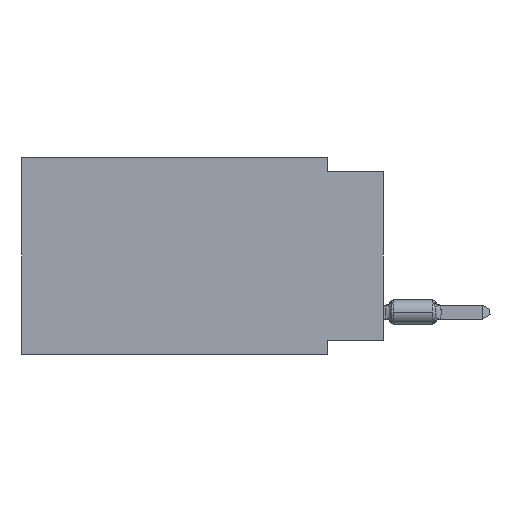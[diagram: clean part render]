
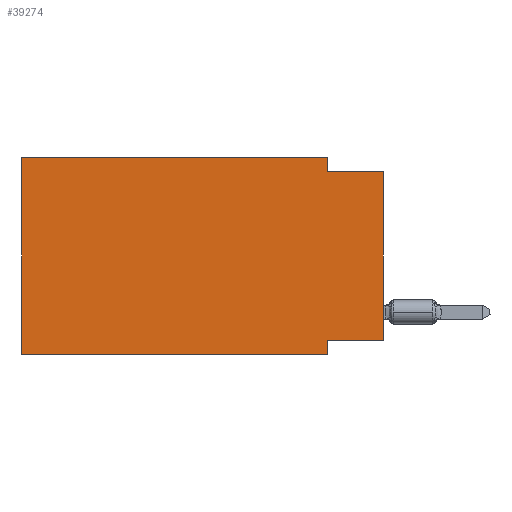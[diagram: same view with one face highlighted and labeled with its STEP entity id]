
A CAD part, left-side view. The second image highlights one B-rep face of the part: STEP entity #39274.
In plain terms, the highlighted planar face has unit normal (-1, 0, 0).
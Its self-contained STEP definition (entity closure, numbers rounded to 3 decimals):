
#858 = ORIENTED_EDGE ( 'NONE', *, *, #37214, .F. ) ;
#1482 = DIRECTION ( 'NONE',  ( 0., 0., 1. ) ) ;
#1789 = CARTESIAN_POINT ( 'NONE',  ( 0., 16.383, 0. ) ) ;
#6985 = EDGE_CURVE ( 'NONE', #53884, #17438, #54228, .T. ) ;
#7641 = VERTEX_POINT ( 'NONE', #52928 ) ;
#9204 = CARTESIAN_POINT ( 'NONE',  ( 0., 0., -8.255 ) ) ;
#9885 = VERTEX_POINT ( 'NONE', #91576 ) ;
#10788 = LINE ( 'NONE', #63070, #44909 ) ;
#12004 = ORIENTED_EDGE ( 'NONE', *, *, #6985, .T. ) ;
#13472 = EDGE_CURVE ( 'NONE', #9885, #17438, #38444, .T. ) ;
#17182 = CARTESIAN_POINT ( 'NONE',  ( 0., 0., -8.255 ) ) ;
#17438 = VERTEX_POINT ( 'NONE', #84281 ) ;
#18834 = CARTESIAN_POINT ( 'NONE',  ( 0., 2.54, -8.89 ) ) ;
#19425 = EDGE_CURVE ( 'NONE', #7641, #9885, #79065, .T. ) ;
#19541 = VERTEX_POINT ( 'NONE', #66823 ) ;
#25354 = FACE_OUTER_BOUND ( 'NONE', #63325, .T. ) ;
#25574 = VECTOR ( 'NONE', #54132, 1000. ) ;
#25694 = CARTESIAN_POINT ( 'NONE',  ( 0., 2.54, -8.255 ) ) ;
#26208 = VECTOR ( 'NONE', #48647, 1000. ) ;
#26300 = ORIENTED_EDGE ( 'NONE', *, *, #95057, .F. ) ;
#26373 = VECTOR ( 'NONE', #78583, 1000. ) ;
#27062 = VECTOR ( 'NONE', #63108, 1000. ) ;
#27740 = CARTESIAN_POINT ( 'NONE',  ( 0., 2.54, 0. ) ) ;
#28400 = EDGE_CURVE ( 'NONE', #70305, #19541, #86717, .T. ) ;
#31174 = LINE ( 'NONE', #67833, #25574 ) ;
#31264 = ORIENTED_EDGE ( 'NONE', *, *, #28400, .F. ) ;
#31972 = ORIENTED_EDGE ( 'NONE', *, *, #13472, .F. ) ;
#33041 = LINE ( 'NONE', #1789, #46982 ) ;
#34318 = VERTEX_POINT ( 'NONE', #50012 ) ;
#37214 = EDGE_CURVE ( 'NONE', #53884, #70305, #84121, .T. ) ;
#38444 = LINE ( 'NONE', #54068, #39547 ) ;
#39274 = ADVANCED_FACE ( 'NONE', ( #25354 ), #60589, .F. ) ;
#39547 = VECTOR ( 'NONE', #47225, 1000. ) ;
#40606 = DIRECTION ( 'NONE',  ( 0., -1., 0. ) ) ;
#42640 = VECTOR ( 'NONE', #1482, 1000. ) ;
#44909 = VECTOR ( 'NONE', #40606, 1000. ) ;
#46982 = VECTOR ( 'NONE', #53563, 1000. ) ;
#47225 = DIRECTION ( 'NONE',  ( 0., -1., 0. ) ) ;
#48647 = DIRECTION ( 'NONE',  ( 0., 0., -1. ) ) ;
#50012 = CARTESIAN_POINT ( 'NONE',  ( 0., 16.383, -8.89 ) ) ;
#50145 = VERTEX_POINT ( 'NONE', #72106 ) ;
#52928 = CARTESIAN_POINT ( 'NONE',  ( 0., 2.54, 0. ) ) ;
#53563 = DIRECTION ( 'NONE',  ( 0., 0., 1. ) ) ;
#53884 = VERTEX_POINT ( 'NONE', #9204 ) ;
#54068 = CARTESIAN_POINT ( 'NONE',  ( 0., 0., -0.635 ) ) ;
#54132 = DIRECTION ( 'NONE',  ( 0., -1., 0. ) ) ;
#54228 = LINE ( 'NONE', #75718, #42640 ) ;
#54691 = DIRECTION ( 'NONE',  ( 1., 0., 0. ) ) ;
#60589 = PLANE ( 'NONE',  #95748 ) ;
#61838 = EDGE_CURVE ( 'NONE', #34318, #50145, #33041, .T. ) ;
#62045 = CARTESIAN_POINT ( 'NONE',  ( 0., 16.383, 0. ) ) ;
#63070 = CARTESIAN_POINT ( 'NONE',  ( 0., 16.383, -8.89 ) ) ;
#63108 = DIRECTION ( 'NONE',  ( 0., 1., 0. ) ) ;
#63325 = EDGE_LOOP ( 'NONE', ( #12004, #31972, #76724, #26300, #66848, #75555, #31264, #858 ) ) ;
#64663 = EDGE_CURVE ( 'NONE', #34318, #19541, #10788, .T. ) ;
#66823 = CARTESIAN_POINT ( 'NONE',  ( 0., 2.54, -8.89 ) ) ;
#66848 = ORIENTED_EDGE ( 'NONE', *, *, #61838, .F. ) ;
#67833 = CARTESIAN_POINT ( 'NONE',  ( 0., 16.383, 0. ) ) ;
#70305 = VERTEX_POINT ( 'NONE', #25694 ) ;
#72106 = CARTESIAN_POINT ( 'NONE',  ( 0., 16.383, 0. ) ) ;
#75555 = ORIENTED_EDGE ( 'NONE', *, *, #64663, .T. ) ;
#75718 = CARTESIAN_POINT ( 'NONE',  ( 0., 0., 0. ) ) ;
#76724 = ORIENTED_EDGE ( 'NONE', *, *, #19425, .F. ) ;
#77156 = DIRECTION ( 'NONE',  ( 0., 0., -1. ) ) ;
#78583 = DIRECTION ( 'NONE',  ( 0., 0., -1. ) ) ;
#79065 = LINE ( 'NONE', #27740, #26373 ) ;
#84121 = LINE ( 'NONE', #17182, #27062 ) ;
#84281 = CARTESIAN_POINT ( 'NONE',  ( 0., 0., -0.635 ) ) ;
#86717 = LINE ( 'NONE', #18834, #26208 ) ;
#91576 = CARTESIAN_POINT ( 'NONE',  ( 0., 2.54, -0.635 ) ) ;
#95057 = EDGE_CURVE ( 'NONE', #50145, #7641, #31174, .T. ) ;
#95748 = AXIS2_PLACEMENT_3D ( 'NONE', #62045, #54691, #77156 ) ;
